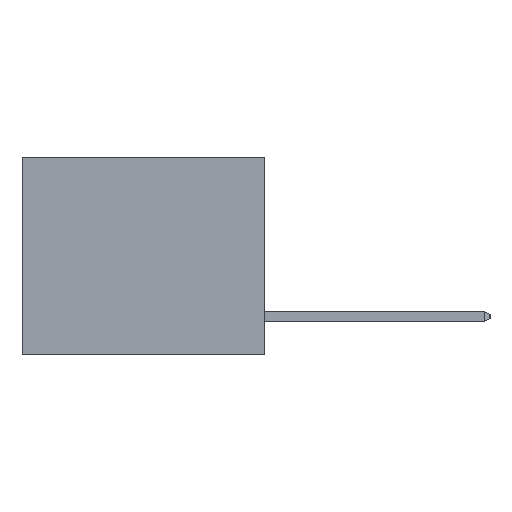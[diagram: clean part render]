
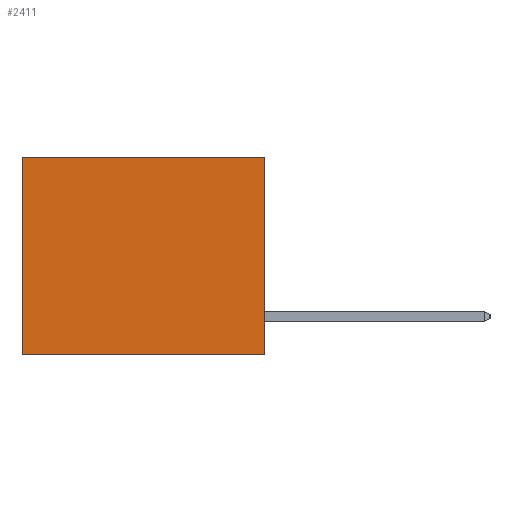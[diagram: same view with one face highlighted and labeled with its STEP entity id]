
A CAD part, left-side view. The second image highlights one B-rep face of the part: STEP entity #2411.
In plain terms, the highlighted planar face has unit normal (-1, 0, 0).
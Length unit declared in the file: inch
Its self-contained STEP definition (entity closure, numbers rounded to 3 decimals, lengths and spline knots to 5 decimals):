
#18 = ORIENTED_EDGE ( 'NONE', *, *, #6506, .F. ) ;
#58 = EDGE_CURVE ( 'NONE', #6327, #1412, #942, .T. ) ;
#647 = CARTESIAN_POINT ( 'NONE',  ( 0.3165, 0., -0.49 ) ) ;
#942 = LINE ( 'NONE', #11404, #5862 ) ;
#1412 = VERTEX_POINT ( 'NONE', #14342 ) ;
#1426 = EDGE_LOOP ( 'NONE', ( #8064, #18, #9322, #10227 ) ) ;
#2162 = CARTESIAN_POINT ( 'NONE',  ( 0.3165, 0., -0.49 ) ) ;
#2411 = ADVANCED_FACE ( 'NONE', ( #12556 ), #3067, .F. ) ;
#2979 = VECTOR ( 'NONE', #8001, 39.37008 ) ;
#3067 = PLANE ( 'NONE',  #12438 ) ;
#3128 = DIRECTION ( 'NONE',  ( 1., 0., 0. ) ) ;
#3187 = CARTESIAN_POINT ( 'NONE',  ( 0.3165, 0.6, -0.49 ) ) ;
#4335 = LINE ( 'NONE', #3187, #2979 ) ;
#5560 = EDGE_CURVE ( 'NONE', #1412, #10033, #4335, .T. ) ;
#5862 = VECTOR ( 'NONE', #12764, 39.37008 ) ;
#6305 = CARTESIAN_POINT ( 'NONE',  ( 0.3165, 0., -0.49 ) ) ;
#6327 = VERTEX_POINT ( 'NONE', #14504 ) ;
#6392 = VECTOR ( 'NONE', #9161, 39.37008 ) ;
#6506 = EDGE_CURVE ( 'NONE', #14682, #10033, #14149, .T. ) ;
#8001 = DIRECTION ( 'NONE',  ( 0., 0., -1. ) ) ;
#8064 = ORIENTED_EDGE ( 'NONE', *, *, #5560, .T. ) ;
#9161 = DIRECTION ( 'NONE',  ( 0., 0., -1. ) ) ;
#9322 = ORIENTED_EDGE ( 'NONE', *, *, #11918, .F. ) ;
#9485 = DIRECTION ( 'NONE',  ( 0., 0., -1. ) ) ;
#10033 = VERTEX_POINT ( 'NONE', #11630 ) ;
#10227 = ORIENTED_EDGE ( 'NONE', *, *, #58, .T. ) ;
#10936 = DIRECTION ( 'NONE',  ( 0., 1., 0. ) ) ;
#11092 = LINE ( 'NONE', #6305, #6392 ) ;
#11404 = CARTESIAN_POINT ( 'NONE',  ( 0.3165, 0., 0. ) ) ;
#11630 = CARTESIAN_POINT ( 'NONE',  ( 0.3165, 0.6, -0.49 ) ) ;
#11918 = EDGE_CURVE ( 'NONE', #6327, #14682, #11092, .T. ) ;
#12438 = AXIS2_PLACEMENT_3D ( 'NONE', #647, #3128, #9485 ) ;
#12556 = FACE_OUTER_BOUND ( 'NONE', #1426, .T. ) ;
#12764 = DIRECTION ( 'NONE',  ( 0., 1., 0. ) ) ;
#14149 = LINE ( 'NONE', #2162, #15317 ) ;
#14342 = CARTESIAN_POINT ( 'NONE',  ( 0.3165, 0.6, 0. ) ) ;
#14504 = CARTESIAN_POINT ( 'NONE',  ( 0.3165, 0., 0. ) ) ;
#14682 = VERTEX_POINT ( 'NONE', #15982 ) ;
#15317 = VECTOR ( 'NONE', #10936, 39.37008 ) ;
#15982 = CARTESIAN_POINT ( 'NONE',  ( 0.3165, 0., -0.49 ) ) ;
